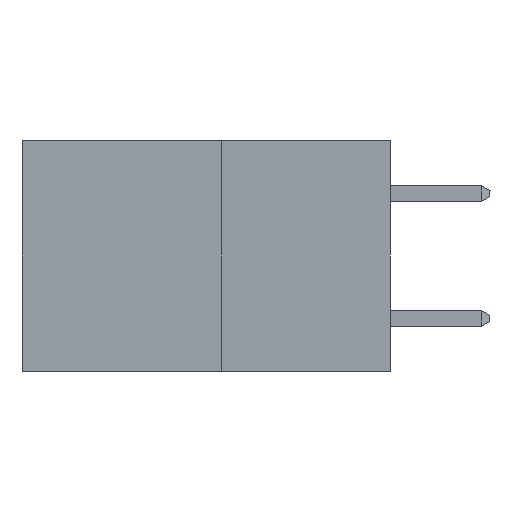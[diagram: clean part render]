
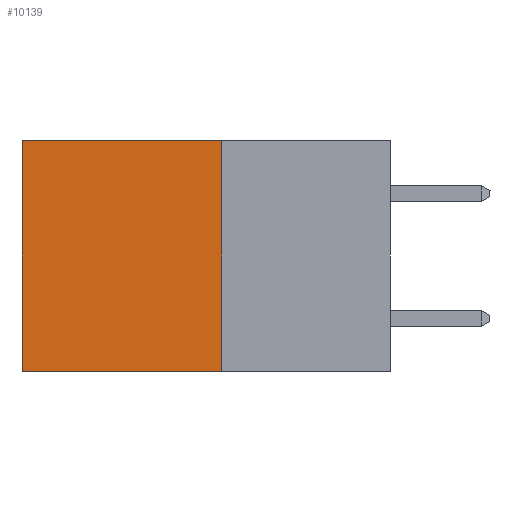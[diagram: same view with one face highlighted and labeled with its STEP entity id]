
A CAD part, left-side view. The second image highlights one B-rep face of the part: STEP entity #10139.
In plain terms, the highlighted planar face has unit normal (-1, 0, 0).
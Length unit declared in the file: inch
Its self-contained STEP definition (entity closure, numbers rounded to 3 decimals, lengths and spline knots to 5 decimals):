
#100 = CARTESIAN_POINT ( 'NONE',  ( 0.277, 0.59, 0. ) ) ;
#413 = EDGE_CURVE ( 'NONE', #1560, #4563, #4992, .T. ) ;
#507 = EDGE_CURVE ( 'NONE', #4563, #3877, #8419, .T. ) ;
#1560 = VERTEX_POINT ( 'NONE', #7458 ) ;
#1822 = DIRECTION ( 'NONE',  ( 0., 1., 0. ) ) ;
#2171 = VECTOR ( 'NONE', #9546, 39.37008 ) ;
#2363 = DIRECTION ( 'NONE',  ( 1., 0., 0. ) ) ;
#3442 = VECTOR ( 'NONE', #6578, 39.37008 ) ;
#3507 = LINE ( 'NONE', #9678, #2171 ) ;
#3877 = VERTEX_POINT ( 'NONE', #7628 ) ;
#3931 = AXIS2_PLACEMENT_3D ( 'NONE', #5431, #2363, #9411 ) ;
#4376 = CARTESIAN_POINT ( 'NONE',  ( 0.277, 0.27, -0.37 ) ) ;
#4563 = VERTEX_POINT ( 'NONE', #8885 ) ;
#4992 = LINE ( 'NONE', #4376, #9904 ) ;
#5124 = VECTOR ( 'NONE', #1822, 39.37008 ) ;
#5265 = EDGE_CURVE ( 'NONE', #1560, #10106, #3507, .T. ) ;
#5431 = CARTESIAN_POINT ( 'NONE',  ( 0.277, 0.27, -0.37 ) ) ;
#5536 = CARTESIAN_POINT ( 'NONE',  ( 0.277, 0.59, -0.37 ) ) ;
#5610 = ORIENTED_EDGE ( 'NONE', *, *, #413, .F. ) ;
#5627 = DIRECTION ( 'NONE',  ( 0., 0., -1. ) ) ;
#6292 = CARTESIAN_POINT ( 'NONE',  ( 0.277, 0.27, -0.37 ) ) ;
#6578 = DIRECTION ( 'NONE',  ( 0., 0., -1. ) ) ;
#7458 = CARTESIAN_POINT ( 'NONE',  ( 0.277, 0.27, 0. ) ) ;
#7628 = CARTESIAN_POINT ( 'NONE',  ( 0.277, 0.59, -0.37 ) ) ;
#7760 = FACE_OUTER_BOUND ( 'NONE', #8931, .T. ) ;
#8419 = LINE ( 'NONE', #6292, #5124 ) ;
#8448 = PLANE ( 'NONE',  #3931 ) ;
#8506 = ORIENTED_EDGE ( 'NONE', *, *, #5265, .T. ) ;
#8885 = CARTESIAN_POINT ( 'NONE',  ( 0.277, 0.27, -0.37 ) ) ;
#8931 = EDGE_LOOP ( 'NONE', ( #11915, #9760, #5610, #8506 ) ) ;
#9411 = DIRECTION ( 'NONE',  ( 0., 0., -1. ) ) ;
#9546 = DIRECTION ( 'NONE',  ( 0., 1., 0. ) ) ;
#9678 = CARTESIAN_POINT ( 'NONE',  ( 0.277, 0.27, 0. ) ) ;
#9760 = ORIENTED_EDGE ( 'NONE', *, *, #507, .F. ) ;
#9904 = VECTOR ( 'NONE', #5627, 39.37008 ) ;
#10106 = VERTEX_POINT ( 'NONE', #100 ) ;
#10139 = ADVANCED_FACE ( 'NONE', ( #7760 ), #8448, .F. ) ;
#11611 = LINE ( 'NONE', #5536, #3442 ) ;
#11657 = EDGE_CURVE ( 'NONE', #10106, #3877, #11611, .T. ) ;
#11915 = ORIENTED_EDGE ( 'NONE', *, *, #11657, .T. ) ;
